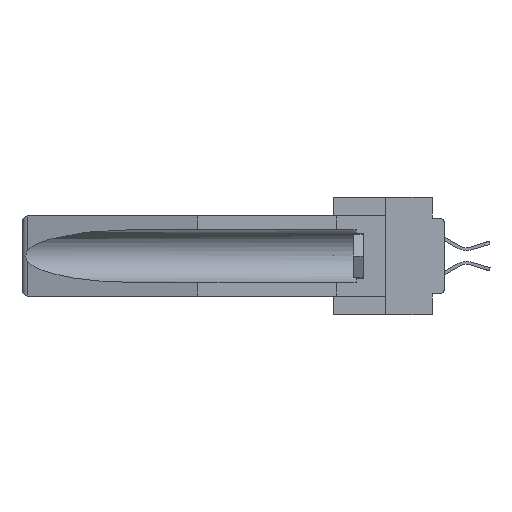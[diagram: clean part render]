
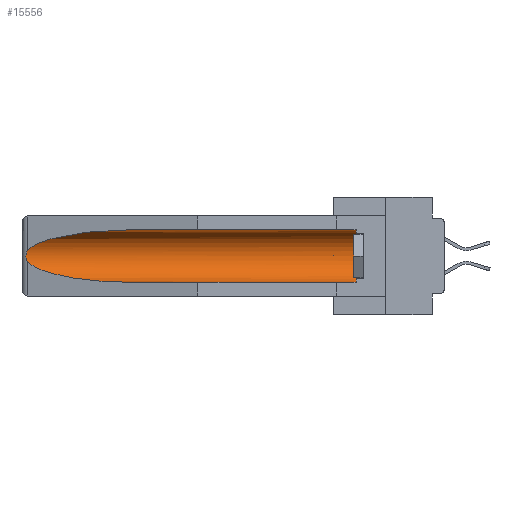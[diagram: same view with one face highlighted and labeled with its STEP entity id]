
A CAD part, left-side view. The second image highlights one B-rep face of the part: STEP entity #15556.
In plain terms, the highlighted cylindrical face has radius 2.857 mm (diameter 5.715 mm), a partial arc.
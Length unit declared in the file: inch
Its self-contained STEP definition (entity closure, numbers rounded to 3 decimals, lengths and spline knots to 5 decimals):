
#78 = VECTOR ( 'NONE', #28594, 39.37008 ) ;
#954 = EDGE_CURVE ( 'NONE', #16941, #2695, #26627, .T. ) ;
#1272 = EDGE_CURVE ( 'NONE', #13595, #19778, #37879, .T. ) ;
#2451 = CARTESIAN_POINT ( 'NONE',  ( 0.26655, 1.53094, -0.18657 ) ) ;
#2643 = CARTESIAN_POINT ( 'NONE',  ( 0.2675, 1.53308, -0.17534 ) ) ;
#2695 = VERTEX_POINT ( 'NONE', #20834 ) ;
#2740 = DIRECTION ( 'NONE',  ( 0., 0., 1. ) ) ;
#4430 = CARTESIAN_POINT ( 'NONE',  ( 0.155, 1.07973, -0.284 ) ) ;
#5110 = FACE_OUTER_BOUND ( 'NONE', #23765, .T. ) ;
#5652 = CARTESIAN_POINT ( 'NONE',  ( 0.26654, 1.53092, -0.15636 ) ) ;
#6744 = ORIENTED_EDGE ( 'NONE', *, *, #35556, .F. ) ;
#7238 = CARTESIAN_POINT ( 'NONE',  ( 0.26537, 1.52718, -0.19328 ) ) ;
#8003 = ORIENTED_EDGE ( 'NONE', *, *, #954, .T. ) ;
#8268 = CARTESIAN_POINT ( 'NONE',  ( 0.26597, 1.5296, -0.19026 ) ) ;
#9202 = CARTESIAN_POINT ( 'NONE',  ( 0.155, 1.07973, -0.059 ) ) ;
#10252 = EDGE_CURVE ( 'NONE', #2695, #14672, #12823, .T. ) ;
#10376 = CARTESIAN_POINT ( 'NONE',  ( 0.155, 1.07973, -0.284 ) ) ;
#11447 = ORIENTED_EDGE ( 'NONE', *, *, #1272, .T. ) ;
#12003 = ORIENTED_EDGE ( 'NONE', *, *, #34689, .T. ) ;
#12823 = LINE ( 'NONE', #16241, #78 ) ;
#13595 = VERTEX_POINT ( 'NONE', #28989 ) ;
#14672 = VERTEX_POINT ( 'NONE', #9202 ) ;
#15556 = ADVANCED_FACE ( 'NONE', ( #5110 ), #20827, .F. ) ;
#16241 = CARTESIAN_POINT ( 'NONE',  ( 0.155, -0.30754, -0.059 ) ) ;
#16941 = VERTEX_POINT ( 'NONE', #36250 ) ;
#17262 = CARTESIAN_POINT ( 'NONE',  ( 0.25451, 1.48313, -0.09465 ) ) ;
#17409 = CARTESIAN_POINT ( 'NONE',  ( 0.155, -0.30754, -0.1715 ) ) ;
#17576 = CARTESIAN_POINT ( 'NONE',  ( 0.26537, 1.52718, -0.14972 ) ) ;
#17965 = CARTESIAN_POINT ( 'NONE',  ( 0.2675, 1.53308, -0.16763 ) ) ;
#18278 = ORIENTED_EDGE ( 'NONE', *, *, #10252, .T. ) ;
#18828 = AXIS2_PLACEMENT_3D ( 'NONE', #33652, #21846, #2740 ) ;
#19739 = CARTESIAN_POINT ( 'NONE',  ( 0.25451, 1.48313, -0.24835 ) ) ;
#19778 = VERTEX_POINT ( 'NONE', #30938 ) ;
#20622 = DIRECTION ( 'NONE',  ( 0., 1., 0. ) ) ;
#20665 = CARTESIAN_POINT ( 'NONE',  ( 0.21114, 1.30732, -0.059 ) ) ;
#20777 = CARTESIAN_POINT ( 'NONE',  ( 0.2673, 1.53269, -0.17917 ) ) ;
#20827 = CYLINDRICAL_SURFACE ( 'NONE', #32008, 0.1125 ) ;
#20834 = CARTESIAN_POINT ( 'NONE',  ( 0.155, 0.126, -0.059 ) ) ;
#21015 = DIRECTION ( 'NONE',  ( 0., 0., 1. ) ) ;
#21846 = DIRECTION ( 'NONE',  ( 0., -1., 0. ) ) ;
#22138 = ORIENTED_EDGE ( 'NONE', *, *, #22153, .T. ) ;
#22153 = EDGE_CURVE ( 'NONE', #19778, #33341, #23152, .T. ) ;
#23152 =( BOUNDED_CURVE ( )  B_SPLINE_CURVE ( 3, ( #7238, #19739, #32140, #4430 ),
 .UNSPECIFIED., .F., .F. ) 
 B_SPLINE_CURVE_WITH_KNOTS ( ( 4, 4 ),
 ( 0.1948, 1.5708 ),
 .UNSPECIFIED. ) 
 CURVE ( )  GEOMETRIC_REPRESENTATION_ITEM ( )  RATIONAL_B_SPLINE_CURVE ( ( 1., 0.848, 0.848, 1. ) ) 
 REPRESENTATION_ITEM ( '' )  );
#23586 = LINE ( 'NONE', #26831, #29733 ) ;
#23732 = CARTESIAN_POINT ( 'NONE',  ( 0.155, 1.07973, -0.059 ) ) ;
#23765 = EDGE_LOOP ( 'NONE', ( #12003, #11447, #22138, #6744, #8003, #18278 ) ) ;
#24427 = CARTESIAN_POINT ( 'NONE',  ( 0.26597, 1.52961, -0.15275 ) ) ;
#26627 = CIRCLE ( 'NONE', #18828, 0.1125 ) ;
#26831 = CARTESIAN_POINT ( 'NONE',  ( 0.155, -0.30754, -0.284 ) ) ;
#27282 = CARTESIAN_POINT ( 'NONE',  ( 0.26537, 1.52718, -0.19328 ) ) ;
#28594 = DIRECTION ( 'NONE',  ( 0., 1., 0. ) ) ;
#28989 = CARTESIAN_POINT ( 'NONE',  ( 0.26537, 1.52718, -0.14972 ) ) ;
#29733 = VECTOR ( 'NONE', #36532, 39.37008 ) ;
#30938 = CARTESIAN_POINT ( 'NONE',  ( 0.26537, 1.52718, -0.19328 ) ) ;
#32008 = AXIS2_PLACEMENT_3D ( 'NONE', #17409, #20622, #21015 ) ;
#32140 = CARTESIAN_POINT ( 'NONE',  ( 0.21114, 1.30732, -0.284 ) ) ;
#33058 = CARTESIAN_POINT ( 'NONE',  ( 0.26537, 1.52718, -0.14972 ) ) ;
#33341 = VERTEX_POINT ( 'NONE', #10376 ) ;
#33652 = CARTESIAN_POINT ( 'NONE',  ( 0.155, 0.126, -0.1715 ) ) ;
#34270 =( BOUNDED_CURVE ( )  B_SPLINE_CURVE ( 3, ( #23732, #20665, #17262, #33058 ),
 .UNSPECIFIED., .F., .F. ) 
 B_SPLINE_CURVE_WITH_KNOTS ( ( 4, 4 ),
 ( 4.71239, 6.08839 ),
 .UNSPECIFIED. ) 
 CURVE ( )  GEOMETRIC_REPRESENTATION_ITEM ( )  RATIONAL_B_SPLINE_CURVE ( ( 1., 0.848, 0.848, 1. ) ) 
 REPRESENTATION_ITEM ( '' )  );
#34689 = EDGE_CURVE ( 'NONE', #14672, #13595, #34270, .T. ) ;
#35556 = EDGE_CURVE ( 'NONE', #16941, #33341, #23586, .T. ) ;
#36250 = CARTESIAN_POINT ( 'NONE',  ( 0.155, 0.126, -0.284 ) ) ;
#36532 = DIRECTION ( 'NONE',  ( 0., 1., 0. ) ) ;
#36780 = CARTESIAN_POINT ( 'NONE',  ( 0.2673, 1.5327, -0.16383 ) ) ;
#37879 = B_SPLINE_CURVE_WITH_KNOTS ( 'NONE', 3,
 ( #17576, #24427, #5652, #36780, #17965, #2643, #20777, #2451, #8268, #27282 ),
 .UNSPECIFIED., .F., .F.,
 ( 4, 2, 2, 2, 4 ),
 ( 0., 0.00029, 0.00058, 0.00087, 0.00117 ),
 .UNSPECIFIED. ) ;
